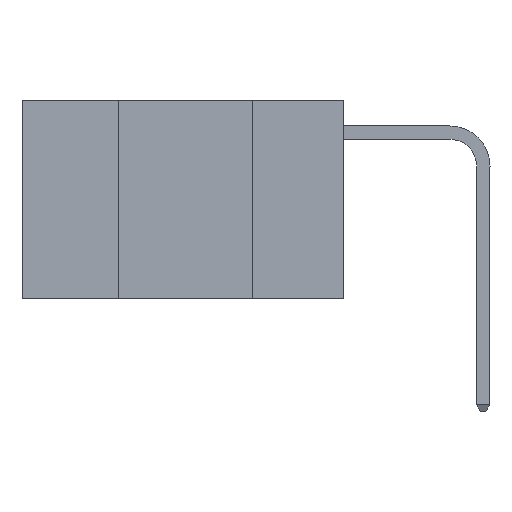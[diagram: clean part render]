
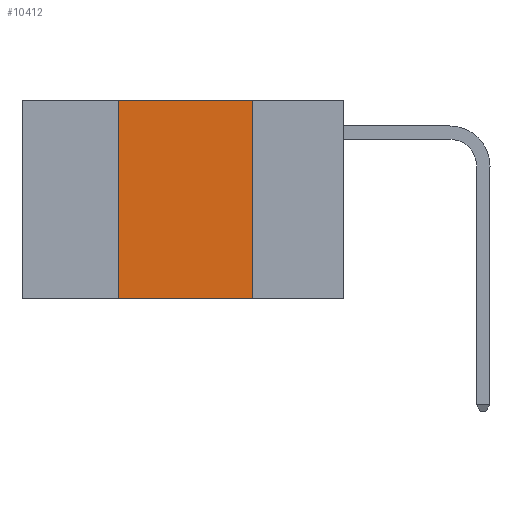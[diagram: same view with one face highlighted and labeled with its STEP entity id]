
A CAD part, left-side view. The second image highlights one B-rep face of the part: STEP entity #10412.
In plain terms, the highlighted planar face has unit normal (-1, 0, 0).
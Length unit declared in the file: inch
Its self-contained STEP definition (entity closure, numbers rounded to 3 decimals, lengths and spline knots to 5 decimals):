
#20 = VECTOR ( 'NONE', #2450, 39.37008 ) ;
#257 = AXIS2_PLACEMENT_3D ( 'NONE', #5373, #7796, #312 ) ;
#312 = DIRECTION ( 'NONE',  ( 0., 0., -1. ) ) ;
#347 = DIRECTION ( 'NONE',  ( 0., -1., 0. ) ) ;
#652 = EDGE_CURVE ( 'NONE', #5702, #6653, #10006, .T. ) ;
#2450 = DIRECTION ( 'NONE',  ( 0., 0., 1. ) ) ;
#3604 = VECTOR ( 'NONE', #347, 39.37008 ) ;
#3770 = CARTESIAN_POINT ( 'NONE',  ( 0., 0.42, 0. ) ) ;
#4033 = DIRECTION ( 'NONE',  ( 0., -1., 0. ) ) ;
#4345 = DIRECTION ( 'NONE',  ( 0., 0., -1. ) ) ;
#5373 = CARTESIAN_POINT ( 'NONE',  ( 0., 0.6, 0. ) ) ;
#5490 = VECTOR ( 'NONE', #4345, 39.37008 ) ;
#5654 = CARTESIAN_POINT ( 'NONE',  ( 0., 0.42, 0. ) ) ;
#5702 = VERTEX_POINT ( 'NONE', #5654 ) ;
#5722 = VERTEX_POINT ( 'NONE', #10473 ) ;
#5958 = ORIENTED_EDGE ( 'NONE', *, *, #15518, .T. ) ;
#6263 = FACE_OUTER_BOUND ( 'NONE', #14859, .T. ) ;
#6589 = PLANE ( 'NONE',  #257 ) ;
#6653 = VERTEX_POINT ( 'NONE', #12188 ) ;
#6658 = EDGE_CURVE ( 'NONE', #10934, #5702, #9901, .T. ) ;
#7796 = DIRECTION ( 'NONE',  ( 1., 0., 0. ) ) ;
#7866 = VECTOR ( 'NONE', #4033, 39.37008 ) ;
#8244 = LINE ( 'NONE', #9994, #7866 ) ;
#9837 = EDGE_CURVE ( 'NONE', #6653, #5722, #15392, .T. ) ;
#9901 = LINE ( 'NONE', #3770, #20 ) ;
#9994 = CARTESIAN_POINT ( 'NONE',  ( 0., 0.6, -0.37 ) ) ;
#10006 = LINE ( 'NONE', #13778, #3604 ) ;
#10412 = ADVANCED_FACE ( 'NONE', ( #6263 ), #6589, .F. ) ;
#10473 = CARTESIAN_POINT ( 'NONE',  ( 0., 0.17, -0.37 ) ) ;
#10934 = VERTEX_POINT ( 'NONE', #13639 ) ;
#12188 = CARTESIAN_POINT ( 'NONE',  ( 0., 0.17, 0. ) ) ;
#13021 = ORIENTED_EDGE ( 'NONE', *, *, #652, .F. ) ;
#13639 = CARTESIAN_POINT ( 'NONE',  ( 0., 0.42, -0.37 ) ) ;
#13778 = CARTESIAN_POINT ( 'NONE',  ( 0., 0.6, 0. ) ) ;
#13955 = ORIENTED_EDGE ( 'NONE', *, *, #6658, .F. ) ;
#14859 = EDGE_LOOP ( 'NONE', ( #15234, #13021, #13955, #5958 ) ) ;
#15079 = CARTESIAN_POINT ( 'NONE',  ( 0., 0.17, 0. ) ) ;
#15234 = ORIENTED_EDGE ( 'NONE', *, *, #9837, .F. ) ;
#15392 = LINE ( 'NONE', #15079, #5490 ) ;
#15518 = EDGE_CURVE ( 'NONE', #10934, #5722, #8244, .T. ) ;
